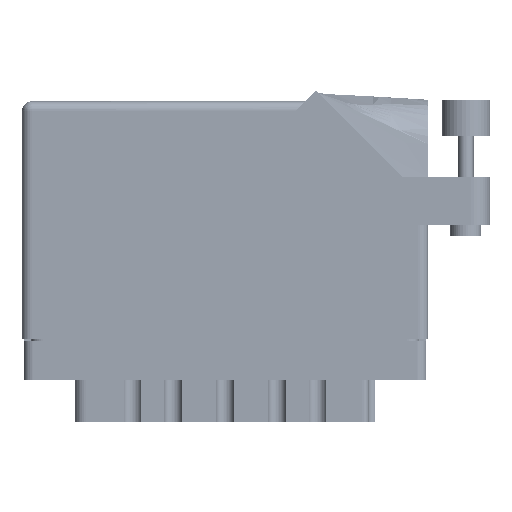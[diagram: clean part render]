
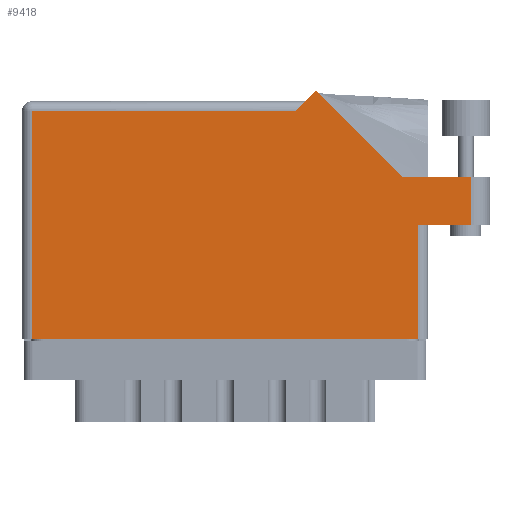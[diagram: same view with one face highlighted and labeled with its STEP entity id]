
A CAD part, front view. The second image highlights one B-rep face of the part: STEP entity #9418.
In plain terms, the highlighted face is planar.
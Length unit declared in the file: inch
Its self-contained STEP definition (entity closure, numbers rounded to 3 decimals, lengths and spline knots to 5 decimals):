
#80 = PLANE ( 'NONE',  #47096 ) ;
#975 = LINE ( 'NONE', #16013, #4900 ) ;
#3005 = CARTESIAN_POINT ( 'NONE',  ( 2.44642, 1.044, 0. ) ) ;
#3812 = ORIENTED_EDGE ( 'NONE', *, *, #24149, .T. ) ;
#4722 = EDGE_CURVE ( 'NONE', #27954, #8125, #52047, .T. ) ;
#4817 = CARTESIAN_POINT ( 'NONE',  ( 0.062, 0., 0. ) ) ;
#4851 = LINE ( 'NONE', #28317, #47648 ) ;
#4900 = VECTOR ( 'NONE', #41017, 39.37008 ) ;
#6141 = VECTOR ( 'NONE', #17284, 39.37008 ) ;
#6767 = LINE ( 'NONE', #24526, #22929 ) ;
#6868 = EDGE_CURVE ( 'NONE', #8125, #35661, #23407, .T. ) ;
#7219 = CARTESIAN_POINT ( 'NONE',  ( 0., 0., 0. ) ) ;
#8086 = CARTESIAN_POINT ( 'NONE',  ( 0., 1.53, 0. ) ) ;
#8125 = VERTEX_POINT ( 'NONE', #18255 ) ;
#8220 = EDGE_CURVE ( 'NONE', #42460, #15736, #10972, .T. ) ;
#8623 = VECTOR ( 'NONE', #48725, 39.37008 ) ;
#8715 = ORIENTED_EDGE ( 'NONE', *, *, #6868, .T. ) ;
#8997 = DIRECTION ( 'NONE',  ( -1., 0., 0. ) ) ;
#9418 = ADVANCED_FACE ( 'NONE', ( #25042 ), #80, .F. ) ;
#9910 = LINE ( 'NONE', #7219, #8623 ) ;
#10972 = LINE ( 'NONE', #3005, #19367 ) ;
#11157 = VERTEX_POINT ( 'NONE', #24981 ) ;
#11830 = ORIENTED_EDGE ( 'NONE', *, *, #8220, .T. ) ;
#12246 = DIRECTION ( 'NONE',  ( -1., 0., 0. ) ) ;
#15730 = ORIENTED_EDGE ( 'NONE', *, *, #34109, .T. ) ;
#15736 = VERTEX_POINT ( 'NONE', #30828 ) ;
#15815 = DIRECTION ( 'NONE',  ( -0.707, -0.707, 0. ) ) ;
#16013 = CARTESIAN_POINT ( 'NONE',  ( 2.612, 0.737, 0. ) ) ;
#17284 = DIRECTION ( 'NONE',  ( 0., 1., 0. ) ) ;
#18255 = CARTESIAN_POINT ( 'NONE',  ( 0.062, 1.468, 0. ) ) ;
#18951 = VECTOR ( 'NONE', #8997, 39.37008 ) ;
#19367 = VECTOR ( 'NONE', #19494, 39.37008 ) ;
#19398 = VERTEX_POINT ( 'NONE', #49702 ) ;
#19405 = ORIENTED_EDGE ( 'NONE', *, *, #47455, .T. ) ;
#19480 = ORIENTED_EDGE ( 'NONE', *, *, #48615, .T. ) ;
#19494 = DIRECTION ( 'NONE',  ( -0.707, 0.707, 0. ) ) ;
#19543 = VECTOR ( 'NONE', #23872, 39.37008 ) ;
#20736 = DIRECTION ( 'NONE',  ( 0., 0., -1. ) ) ;
#21453 = CARTESIAN_POINT ( 'NONE',  ( 0., 1.468, 0. ) ) ;
#21556 = EDGE_LOOP ( 'NONE', ( #19405, #3812, #29786, #11830, #19480, #21786, #8715, #29726, #15730 ) ) ;
#21786 = ORIENTED_EDGE ( 'NONE', *, *, #4722, .T. ) ;
#22929 = VECTOR ( 'NONE', #28368, 39.37008 ) ;
#23407 = LINE ( 'NONE', #30039, #19543 ) ;
#23872 = DIRECTION ( 'NONE',  ( 0., -1., 0. ) ) ;
#23964 = CARTESIAN_POINT ( 'NONE',  ( 2.887, 1.044, 0. ) ) ;
#24149 = EDGE_CURVE ( 'NONE', #19398, #53127, #44993, .T. ) ;
#24176 = CARTESIAN_POINT ( 'NONE',  ( 2.887, 1.044, 0. ) ) ;
#24526 = CARTESIAN_POINT ( 'NONE',  ( 3.012, 1.044, 0. ) ) ;
#24623 = EDGE_CURVE ( 'NONE', #35661, #11157, #9910, .T. ) ;
#24981 = CARTESIAN_POINT ( 'NONE',  ( 2.55, 0., 0. ) ) ;
#25042 = FACE_OUTER_BOUND ( 'NONE', #21556, .T. ) ;
#26790 = VECTOR ( 'NONE', #53007, 39.37008 ) ;
#27954 = VERTEX_POINT ( 'NONE', #52144 ) ;
#28317 = CARTESIAN_POINT ( 'NONE',  ( 1.819, 1.53, 0. ) ) ;
#28368 = DIRECTION ( 'NONE',  ( -1., 0., 0. ) ) ;
#29726 = ORIENTED_EDGE ( 'NONE', *, *, #24623, .T. ) ;
#29786 = ORIENTED_EDGE ( 'NONE', *, *, #34037, .T. ) ;
#30039 = CARTESIAN_POINT ( 'NONE',  ( 0.062, 0., 0. ) ) ;
#30828 = CARTESIAN_POINT ( 'NONE',  ( 1.88971, 1.60071, 0. ) ) ;
#34037 = EDGE_CURVE ( 'NONE', #53127, #42460, #6767, .T. ) ;
#34109 = EDGE_CURVE ( 'NONE', #11157, #36530, #42444, .T. ) ;
#35661 = VERTEX_POINT ( 'NONE', #4817 ) ;
#36530 = VERTEX_POINT ( 'NONE', #44220 ) ;
#37411 = CARTESIAN_POINT ( 'NONE',  ( 2.44642, 1.044, 0. ) ) ;
#41017 = DIRECTION ( 'NONE',  ( 1., 0., 0. ) ) ;
#42444 = LINE ( 'NONE', #50451, #6141 ) ;
#42460 = VERTEX_POINT ( 'NONE', #37411 ) ;
#44220 = CARTESIAN_POINT ( 'NONE',  ( 2.55, 0.737, 0. ) ) ;
#44993 = LINE ( 'NONE', #23964, #26790 ) ;
#47096 = AXIS2_PLACEMENT_3D ( 'NONE', #8086, #20736, #12246 ) ;
#47455 = EDGE_CURVE ( 'NONE', #36530, #19398, #975, .T. ) ;
#47648 = VECTOR ( 'NONE', #15815, 39.37008 ) ;
#48615 = EDGE_CURVE ( 'NONE', #15736, #27954, #4851, .T. ) ;
#48725 = DIRECTION ( 'NONE',  ( 1., 0., 0. ) ) ;
#49702 = CARTESIAN_POINT ( 'NONE',  ( 2.887, 0.737, 0. ) ) ;
#50451 = CARTESIAN_POINT ( 'NONE',  ( 2.55, 0.737, 0. ) ) ;
#52047 = LINE ( 'NONE', #21453, #18951 ) ;
#52144 = CARTESIAN_POINT ( 'NONE',  ( 1.757, 1.468, 0. ) ) ;
#53007 = DIRECTION ( 'NONE',  ( 0., 1., 0. ) ) ;
#53127 = VERTEX_POINT ( 'NONE', #24176 ) ;
